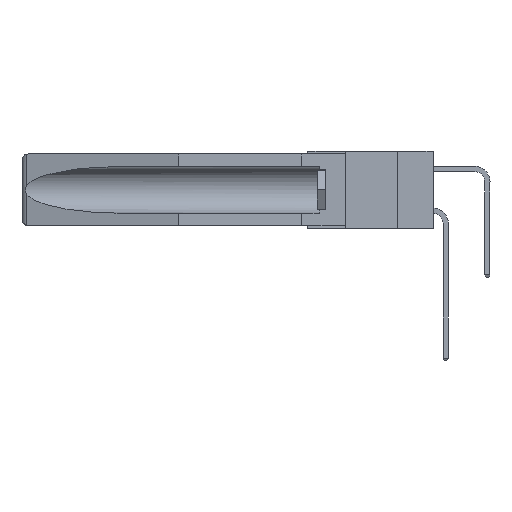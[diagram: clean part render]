
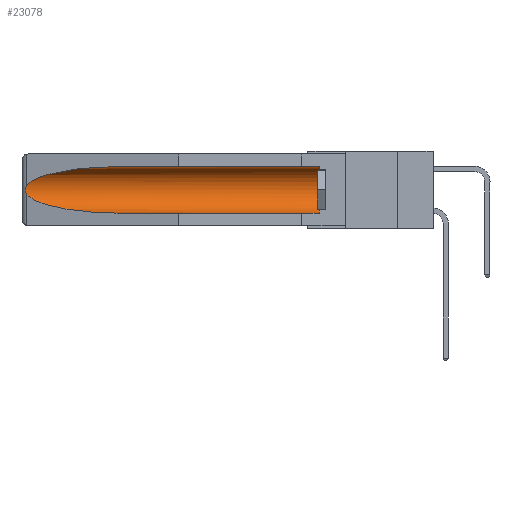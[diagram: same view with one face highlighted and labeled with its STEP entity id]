
A CAD part, left-side view. The second image highlights one B-rep face of the part: STEP entity #23078.
In plain terms, the highlighted cylindrical face has radius 2.857 mm (diameter 5.715 mm), a partial arc.
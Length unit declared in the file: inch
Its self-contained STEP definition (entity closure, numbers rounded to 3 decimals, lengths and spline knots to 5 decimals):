
#615 = CARTESIAN_POINT ( 'NONE',  ( 0.155, 1.07973, -0.284 ) ) ;
#956 = CARTESIAN_POINT ( 'NONE',  ( 0.26537, 1.52718, -0.14972 ) ) ;
#1186 = CARTESIAN_POINT ( 'NONE',  ( 0.155, 0.126, -0.1715 ) ) ;
#2428 = CARTESIAN_POINT ( 'NONE',  ( 0.155, -0.30754, -0.059 ) ) ;
#3257 = ORIENTED_EDGE ( 'NONE', *, *, #27134, .T. ) ;
#3297 = CARTESIAN_POINT ( 'NONE',  ( 0.26537, 1.52718, -0.19328 ) ) ;
#4120 = VECTOR ( 'NONE', #14074, 39.37008 ) ;
#4139 = CARTESIAN_POINT ( 'NONE',  ( 0.26537, 1.52718, -0.19328 ) ) ;
#4418 = EDGE_CURVE ( 'NONE', #22669, #18269, #5267, .T. ) ;
#4918 = CARTESIAN_POINT ( 'NONE',  ( 0.26537, 1.52718, -0.14972 ) ) ;
#5267 = LINE ( 'NONE', #31118, #4120 ) ;
#6028 = CARTESIAN_POINT ( 'NONE',  ( 0.26597, 1.5296, -0.19026 ) ) ;
#6491 = DIRECTION ( 'NONE',  ( 0., 1., 0. ) ) ;
#7207 = EDGE_CURVE ( 'NONE', #22669, #27784, #11958, .T. ) ;
#7216 =( BOUNDED_CURVE ( )  B_SPLINE_CURVE ( 3, ( #30416, #16156, #28509, #4918 ),
 .UNSPECIFIED., .F., .F. ) 
 B_SPLINE_CURVE_WITH_KNOTS ( ( 4, 4 ),
 ( 4.71239, 6.08839 ),
 .UNSPECIFIED. ) 
 CURVE ( )  GEOMETRIC_REPRESENTATION_ITEM ( )  RATIONAL_B_SPLINE_CURVE ( ( 1., 0.848, 0.848, 1. ) ) 
 REPRESENTATION_ITEM ( '' )  );
#7833 = EDGE_CURVE ( 'NONE', #27784, #11393, #9272, .T. ) ;
#8935 = DIRECTION ( 'NONE',  ( 0., 0., 1. ) ) ;
#9272 = LINE ( 'NONE', #2428, #22769 ) ;
#9345 = ORIENTED_EDGE ( 'NONE', *, *, #7833, .T. ) ;
#9455 = CARTESIAN_POINT ( 'NONE',  ( 0.155, 0.126, -0.059 ) ) ;
#10660 = CARTESIAN_POINT ( 'NONE',  ( 0.25451, 1.48313, -0.24835 ) ) ;
#10674 =( BOUNDED_CURVE ( )  B_SPLINE_CURVE ( 3, ( #15068, #10660, #12987, #615 ),
 .UNSPECIFIED., .F., .F. ) 
 B_SPLINE_CURVE_WITH_KNOTS ( ( 4, 4 ),
 ( 0.1948, 1.5708 ),
 .UNSPECIFIED. ) 
 CURVE ( )  GEOMETRIC_REPRESENTATION_ITEM ( )  RATIONAL_B_SPLINE_CURVE ( ( 1., 0.848, 0.848, 1. ) ) 
 REPRESENTATION_ITEM ( '' )  );
#11054 = CARTESIAN_POINT ( 'NONE',  ( 0.26537, 1.52718, -0.14972 ) ) ;
#11069 = CARTESIAN_POINT ( 'NONE',  ( 0.155, 1.07973, -0.284 ) ) ;
#11393 = VERTEX_POINT ( 'NONE', #27101 ) ;
#11958 = CIRCLE ( 'NONE', #16120, 0.1125 ) ;
#12675 = VERTEX_POINT ( 'NONE', #11054 ) ;
#12987 = CARTESIAN_POINT ( 'NONE',  ( 0.21114, 1.30732, -0.284 ) ) ;
#13208 = CARTESIAN_POINT ( 'NONE',  ( 0.2673, 1.53269, -0.17917 ) ) ;
#13456 = CARTESIAN_POINT ( 'NONE',  ( 0.155, -0.30754, -0.1715 ) ) ;
#13676 = ORIENTED_EDGE ( 'NONE', *, *, #15069, .T. ) ;
#14074 = DIRECTION ( 'NONE',  ( 0., 1., 0. ) ) ;
#15068 = CARTESIAN_POINT ( 'NONE',  ( 0.26537, 1.52718, -0.19328 ) ) ;
#15069 = EDGE_CURVE ( 'NONE', #11393, #12675, #7216, .T. ) ;
#15595 = CARTESIAN_POINT ( 'NONE',  ( 0.26655, 1.53094, -0.18657 ) ) ;
#16120 = AXIS2_PLACEMENT_3D ( 'NONE', #1186, #18240, #20642 ) ;
#16156 = CARTESIAN_POINT ( 'NONE',  ( 0.21114, 1.30732, -0.059 ) ) ;
#17588 = EDGE_LOOP ( 'NONE', ( #13676, #28258, #3257, #29678, #19017, #9345 ) ) ;
#17606 = EDGE_CURVE ( 'NONE', #12675, #26683, #20462, .T. ) ;
#17717 = CARTESIAN_POINT ( 'NONE',  ( 0.2675, 1.53308, -0.17534 ) ) ;
#18240 = DIRECTION ( 'NONE',  ( 0., -1., 0. ) ) ;
#18269 = VERTEX_POINT ( 'NONE', #11069 ) ;
#19017 = ORIENTED_EDGE ( 'NONE', *, *, #7207, .T. ) ;
#20462 = B_SPLINE_CURVE_WITH_KNOTS ( 'NONE', 3,
 ( #956, #22839, #29636, #27433, #22532, #17717, #13208, #15595, #6028, #3297 ),
 .UNSPECIFIED., .F., .F.,
 ( 4, 2, 2, 2, 4 ),
 ( 0., 0.00029, 0.00058, 0.00087, 0.00117 ),
 .UNSPECIFIED. ) ;
#20642 = DIRECTION ( 'NONE',  ( 0., 0., 1. ) ) ;
#22532 = CARTESIAN_POINT ( 'NONE',  ( 0.2675, 1.53308, -0.16763 ) ) ;
#22542 = FACE_OUTER_BOUND ( 'NONE', #17588, .T. ) ;
#22669 = VERTEX_POINT ( 'NONE', #27616 ) ;
#22769 = VECTOR ( 'NONE', #28683, 39.37008 ) ;
#22839 = CARTESIAN_POINT ( 'NONE',  ( 0.26597, 1.52961, -0.15275 ) ) ;
#23078 = ADVANCED_FACE ( 'NONE', ( #22542 ), #27916, .F. ) ;
#26683 = VERTEX_POINT ( 'NONE', #4139 ) ;
#27101 = CARTESIAN_POINT ( 'NONE',  ( 0.155, 1.07973, -0.059 ) ) ;
#27134 = EDGE_CURVE ( 'NONE', #26683, #18269, #10674, .T. ) ;
#27433 = CARTESIAN_POINT ( 'NONE',  ( 0.2673, 1.5327, -0.16383 ) ) ;
#27616 = CARTESIAN_POINT ( 'NONE',  ( 0.155, 0.126, -0.284 ) ) ;
#27632 = AXIS2_PLACEMENT_3D ( 'NONE', #13456, #6491, #8935 ) ;
#27784 = VERTEX_POINT ( 'NONE', #9455 ) ;
#27916 = CYLINDRICAL_SURFACE ( 'NONE', #27632, 0.1125 ) ;
#28258 = ORIENTED_EDGE ( 'NONE', *, *, #17606, .T. ) ;
#28509 = CARTESIAN_POINT ( 'NONE',  ( 0.25451, 1.48313, -0.09465 ) ) ;
#28683 = DIRECTION ( 'NONE',  ( 0., 1., 0. ) ) ;
#29636 = CARTESIAN_POINT ( 'NONE',  ( 0.26654, 1.53092, -0.15636 ) ) ;
#29678 = ORIENTED_EDGE ( 'NONE', *, *, #4418, .F. ) ;
#30416 = CARTESIAN_POINT ( 'NONE',  ( 0.155, 1.07973, -0.059 ) ) ;
#31118 = CARTESIAN_POINT ( 'NONE',  ( 0.155, -0.30754, -0.284 ) ) ;
